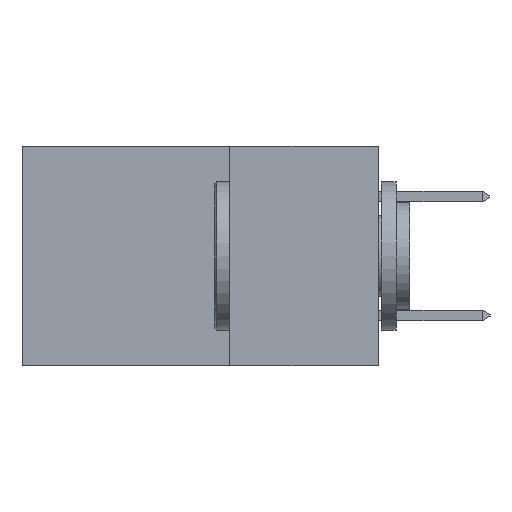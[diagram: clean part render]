
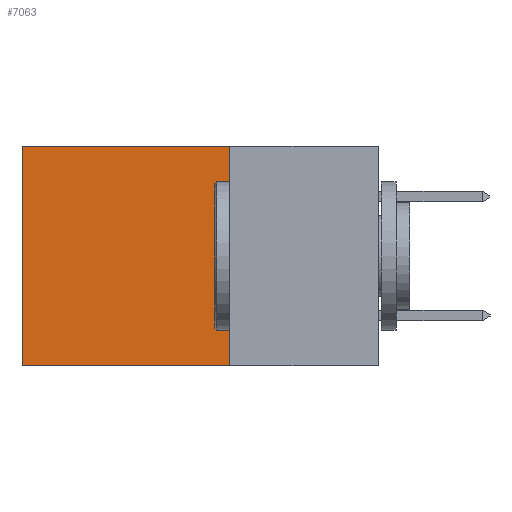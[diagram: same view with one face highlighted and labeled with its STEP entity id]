
A CAD part, left-side view. The second image highlights one B-rep face of the part: STEP entity #7063.
In plain terms, the highlighted planar face has unit normal (-1, 0, 0).
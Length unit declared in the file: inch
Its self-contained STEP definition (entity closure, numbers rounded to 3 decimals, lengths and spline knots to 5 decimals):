
#35 = CARTESIAN_POINT ( 'NONE',  ( 0.2615, 0.25, -0.37 ) ) ;
#965 = EDGE_CURVE ( 'NONE', #1561, #1291, #5622, .T. ) ;
#1280 = ORIENTED_EDGE ( 'NONE', *, *, #7629, .T. ) ;
#1291 = VERTEX_POINT ( 'NONE', #6353 ) ;
#1310 = EDGE_CURVE ( 'NONE', #1561, #9180, #7486, .T. ) ;
#1499 = VECTOR ( 'NONE', #7530, 39.37008 ) ;
#1561 = VERTEX_POINT ( 'NONE', #4875 ) ;
#1721 = CARTESIAN_POINT ( 'NONE',  ( 0.2615, 0.6, -0.37 ) ) ;
#1810 = CARTESIAN_POINT ( 'NONE',  ( 0.2615, 0.6, -0.37 ) ) ;
#2902 = CARTESIAN_POINT ( 'NONE',  ( 0.2615, 0.6, 0. ) ) ;
#3181 = LINE ( 'NONE', #1721, #6955 ) ;
#3872 = EDGE_LOOP ( 'NONE', ( #1280, #6027, #9156, #5558 ) ) ;
#3990 = PLANE ( 'NONE',  #6823 ) ;
#4039 = DIRECTION ( 'NONE',  ( 0., 0., -1. ) ) ;
#4651 = LINE ( 'NONE', #35, #8183 ) ;
#4720 = DIRECTION ( 'NONE',  ( 1., 0., 0. ) ) ;
#4875 = CARTESIAN_POINT ( 'NONE',  ( 0.2615, 0.25, 0. ) ) ;
#5436 = VERTEX_POINT ( 'NONE', #1810 ) ;
#5558 = ORIENTED_EDGE ( 'NONE', *, *, #1310, .T. ) ;
#5622 = LINE ( 'NONE', #6357, #9210 ) ;
#6027 = ORIENTED_EDGE ( 'NONE', *, *, #6123, .F. ) ;
#6123 = EDGE_CURVE ( 'NONE', #1291, #5436, #4651, .T. ) ;
#6353 = CARTESIAN_POINT ( 'NONE',  ( 0.2615, 0.25, -0.37 ) ) ;
#6357 = CARTESIAN_POINT ( 'NONE',  ( 0.2615, 0.25, -0.37 ) ) ;
#6823 = AXIS2_PLACEMENT_3D ( 'NONE', #8436, #4720, #9811 ) ;
#6955 = VECTOR ( 'NONE', #6966, 39.37008 ) ;
#6966 = DIRECTION ( 'NONE',  ( 0., 0., -1. ) ) ;
#7063 = ADVANCED_FACE ( 'NONE', ( #8381 ), #3990, .F. ) ;
#7486 = LINE ( 'NONE', #7601, #1499 ) ;
#7530 = DIRECTION ( 'NONE',  ( 0., 1., 0. ) ) ;
#7601 = CARTESIAN_POINT ( 'NONE',  ( 0.2615, 0.25, 0. ) ) ;
#7629 = EDGE_CURVE ( 'NONE', #9180, #5436, #3181, .T. ) ;
#8183 = VECTOR ( 'NONE', #8488, 39.37008 ) ;
#8381 = FACE_OUTER_BOUND ( 'NONE', #3872, .T. ) ;
#8436 = CARTESIAN_POINT ( 'NONE',  ( 0.2615, 0.25, -0.37 ) ) ;
#8488 = DIRECTION ( 'NONE',  ( 0., 1., 0. ) ) ;
#9156 = ORIENTED_EDGE ( 'NONE', *, *, #965, .F. ) ;
#9180 = VERTEX_POINT ( 'NONE', #2902 ) ;
#9210 = VECTOR ( 'NONE', #4039, 39.37008 ) ;
#9811 = DIRECTION ( 'NONE',  ( 0., 0., -1. ) ) ;
